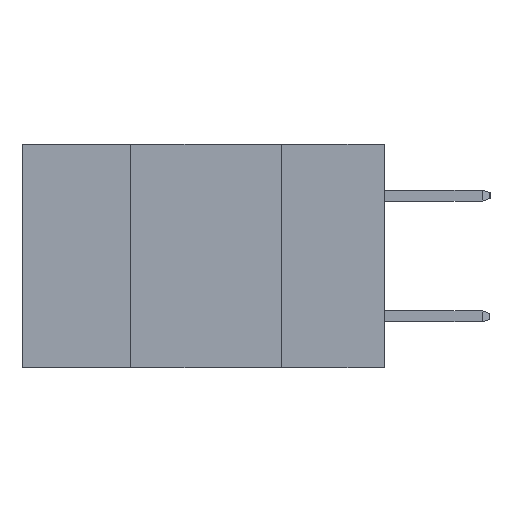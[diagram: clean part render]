
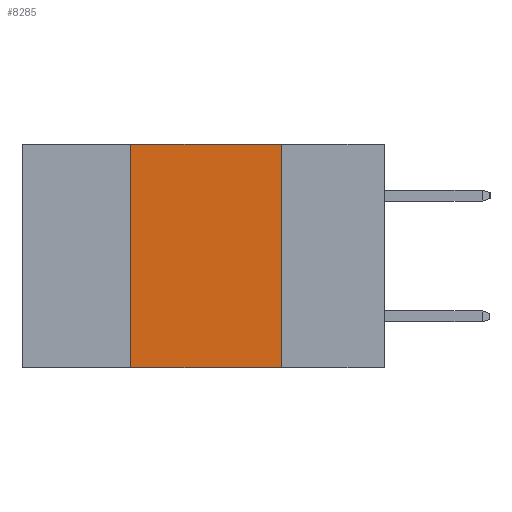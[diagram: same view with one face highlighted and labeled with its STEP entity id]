
A CAD part, left-side view. The second image highlights one B-rep face of the part: STEP entity #8285.
In plain terms, the highlighted planar face has unit normal (-1, 0, 0).
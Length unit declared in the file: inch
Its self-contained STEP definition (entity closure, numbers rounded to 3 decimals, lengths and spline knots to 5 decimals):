
#104 = ORIENTED_EDGE ( 'NONE', *, *, #8883, .F. ) ;
#125 = DIRECTION ( 'NONE',  ( 0., -1., 0. ) ) ;
#568 = CARTESIAN_POINT ( 'NONE',  ( 0., 0.17, 0. ) ) ;
#778 = VERTEX_POINT ( 'NONE', #8817 ) ;
#1361 = LINE ( 'NONE', #568, #5403 ) ;
#1476 = DIRECTION ( 'NONE',  ( 0., 0., -1. ) ) ;
#1627 = ORIENTED_EDGE ( 'NONE', *, *, #3079, .T. ) ;
#1629 = DIRECTION ( 'NONE',  ( 0., 0., 1. ) ) ;
#2150 = CARTESIAN_POINT ( 'NONE',  ( 0., 0.42, -0.37 ) ) ;
#2422 = ORIENTED_EDGE ( 'NONE', *, *, #6430, .F. ) ;
#2997 = VERTEX_POINT ( 'NONE', #7333 ) ;
#3079 = EDGE_CURVE ( 'NONE', #4754, #778, #8522, .T. ) ;
#3764 = PLANE ( 'NONE',  #8171 ) ;
#4093 = EDGE_CURVE ( 'NONE', #4754, #2997, #7775, .T. ) ;
#4377 = VECTOR ( 'NONE', #125, 39.37008 ) ;
#4751 = FACE_OUTER_BOUND ( 'NONE', #8578, .T. ) ;
#4754 = VERTEX_POINT ( 'NONE', #2150 ) ;
#4867 = VECTOR ( 'NONE', #8376, 39.37008 ) ;
#5343 = LINE ( 'NONE', #8434, #4867 ) ;
#5403 = VECTOR ( 'NONE', #1476, 39.37008 ) ;
#5627 = CARTESIAN_POINT ( 'NONE',  ( 0., 0.17, 0. ) ) ;
#5705 = VECTOR ( 'NONE', #1629, 39.37008 ) ;
#6391 = VERTEX_POINT ( 'NONE', #5627 ) ;
#6430 = EDGE_CURVE ( 'NONE', #6391, #778, #1361, .T. ) ;
#7333 = CARTESIAN_POINT ( 'NONE',  ( 0., 0.42, 0. ) ) ;
#7357 = ORIENTED_EDGE ( 'NONE', *, *, #4093, .F. ) ;
#7775 = LINE ( 'NONE', #9979, #5705 ) ;
#8171 = AXIS2_PLACEMENT_3D ( 'NONE', #9164, #8672, #9800 ) ;
#8285 = ADVANCED_FACE ( 'NONE', ( #4751 ), #3764, .F. ) ;
#8376 = DIRECTION ( 'NONE',  ( 0., -1., 0. ) ) ;
#8434 = CARTESIAN_POINT ( 'NONE',  ( 0., 0.6, 0. ) ) ;
#8522 = LINE ( 'NONE', #8760, #4377 ) ;
#8578 = EDGE_LOOP ( 'NONE', ( #2422, #104, #7357, #1627 ) ) ;
#8672 = DIRECTION ( 'NONE',  ( 1., 0., 0. ) ) ;
#8760 = CARTESIAN_POINT ( 'NONE',  ( 0., 0.6, -0.37 ) ) ;
#8817 = CARTESIAN_POINT ( 'NONE',  ( 0., 0.17, -0.37 ) ) ;
#8883 = EDGE_CURVE ( 'NONE', #2997, #6391, #5343, .T. ) ;
#9164 = CARTESIAN_POINT ( 'NONE',  ( 0., 0.6, 0. ) ) ;
#9800 = DIRECTION ( 'NONE',  ( 0., 0., -1. ) ) ;
#9979 = CARTESIAN_POINT ( 'NONE',  ( 0., 0.42, 0. ) ) ;
